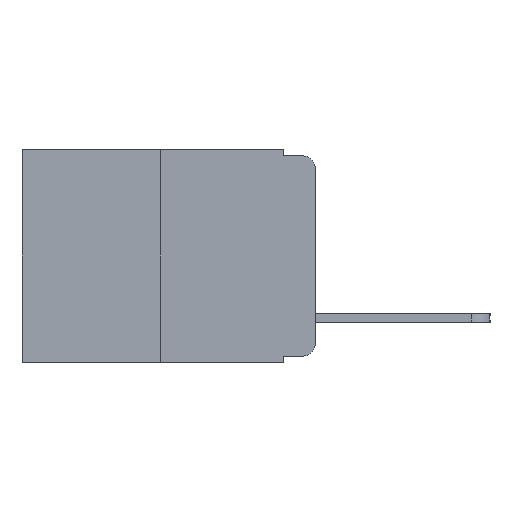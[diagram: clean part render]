
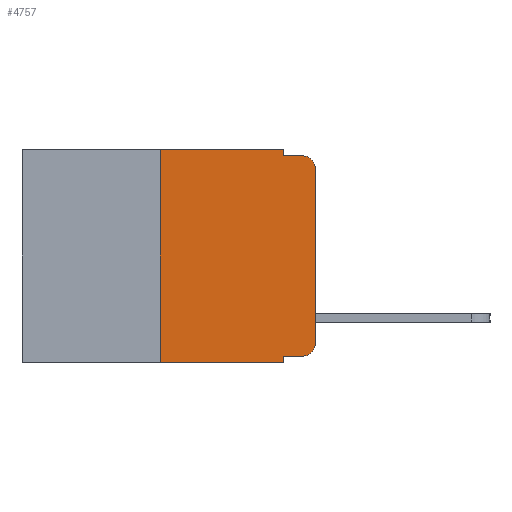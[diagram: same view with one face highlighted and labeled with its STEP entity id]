
A CAD part, left-side view. The second image highlights one B-rep face of the part: STEP entity #4757.
In plain terms, the highlighted planar face has unit normal (-1, 0, 0).
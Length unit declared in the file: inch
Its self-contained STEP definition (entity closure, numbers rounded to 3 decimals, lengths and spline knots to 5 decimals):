
#503 = VERTEX_POINT ( 'NONE', #1208 ) ;
#632 = DIRECTION ( 'NONE',  ( 0., 0., -1. ) ) ;
#1208 = CARTESIAN_POINT ( 'NONE',  ( 0., 0., -0.313 ) ) ;
#1464 = DIRECTION ( 'NONE',  ( 0., -1., 0. ) ) ;
#1510 = VECTOR ( 'NONE', #7378, 39.37008 ) ;
#1657 = LINE ( 'NONE', #4870, #13561 ) ;
#1667 = AXIS2_PLACEMENT_3D ( 'NONE', #4484, #5645, #13725 ) ;
#1835 = AXIS2_PLACEMENT_3D ( 'NONE', #14450, #7539, #632 ) ;
#2133 = CIRCLE ( 'NONE', #3770, 0.02 ) ;
#2329 = EDGE_CURVE ( 'NONE', #2758, #6144, #1657, .T. ) ;
#2381 = VECTOR ( 'NONE', #5413, 39.37008 ) ;
#2434 = EDGE_CURVE ( 'NONE', #12145, #6104, #10714, .T. ) ;
#2583 = EDGE_CURVE ( 'NONE', #11975, #2758, #11249, .T. ) ;
#2726 = ORIENTED_EDGE ( 'NONE', *, *, #2434, .F. ) ;
#2758 = VERTEX_POINT ( 'NONE', #14878 ) ;
#2900 = VERTEX_POINT ( 'NONE', #10627 ) ;
#3063 = EDGE_CURVE ( 'NONE', #3252, #11975, #4716, .T. ) ;
#3070 = EDGE_LOOP ( 'NONE', ( #3589, #12847, #13886, #4369, #11630, #12729, #10726, #2726, #9956, #5263 ) ) ;
#3252 = VERTEX_POINT ( 'NONE', #11225 ) ;
#3296 = CARTESIAN_POINT ( 'NONE',  ( 0., 0.051, -0.333 ) ) ;
#3589 = ORIENTED_EDGE ( 'NONE', *, *, #11612, .T. ) ;
#3770 = AXIS2_PLACEMENT_3D ( 'NONE', #13315, #6368, #14443 ) ;
#3987 = CARTESIAN_POINT ( 'NONE',  ( 0., 0.473, 0. ) ) ;
#4195 = EDGE_CURVE ( 'NONE', #12145, #2900, #8632, .T. ) ;
#4244 = CARTESIAN_POINT ( 'NONE',  ( 0., 0.051, 0. ) ) ;
#4254 = EDGE_CURVE ( 'NONE', #2900, #503, #2133, .T. ) ;
#4369 = ORIENTED_EDGE ( 'NONE', *, *, #2583, .F. ) ;
#4417 = EDGE_CURVE ( 'NONE', #7759, #6104, #14564, .T. ) ;
#4463 = FACE_OUTER_BOUND ( 'NONE', #3070, .T. ) ;
#4484 = CARTESIAN_POINT ( 'NONE',  ( 0., 0.473, 0. ) ) ;
#4716 = LINE ( 'NONE', #3987, #13564 ) ;
#4757 = ADVANCED_FACE ( 'NONE', ( #4463 ), #11435, .F. ) ;
#4759 = CARTESIAN_POINT ( 'NONE',  ( 0., 0.051, -0.343 ) ) ;
#4870 = CARTESIAN_POINT ( 'NONE',  ( 0., 0.051, -0.01 ) ) ;
#4887 = CARTESIAN_POINT ( 'NONE',  ( 0., 0.25, 0. ) ) ;
#4995 = EDGE_CURVE ( 'NONE', #7759, #3252, #12805, .T. ) ;
#5147 = DIRECTION ( 'NONE',  ( 0., -1., 0. ) ) ;
#5263 = ORIENTED_EDGE ( 'NONE', *, *, #4254, .T. ) ;
#5275 = CARTESIAN_POINT ( 'NONE',  ( 0., 0.051, 0. ) ) ;
#5372 = VECTOR ( 'NONE', #14731, 39.37008 ) ;
#5413 = DIRECTION ( 'NONE',  ( 0., 0., -1. ) ) ;
#5645 = DIRECTION ( 'NONE',  ( 1., 0., 0. ) ) ;
#5792 = DIRECTION ( 'NONE',  ( 0., 0., 1. ) ) ;
#6104 = VERTEX_POINT ( 'NONE', #4759 ) ;
#6144 = VERTEX_POINT ( 'NONE', #7124 ) ;
#6368 = DIRECTION ( 'NONE',  ( -1., 0., 0. ) ) ;
#7124 = CARTESIAN_POINT ( 'NONE',  ( 0., 0.02, -0.01 ) ) ;
#7378 = DIRECTION ( 'NONE',  ( 0., 0., -1. ) ) ;
#7539 = DIRECTION ( 'NONE',  ( -1., 0., 0. ) ) ;
#7759 = VERTEX_POINT ( 'NONE', #7926 ) ;
#7835 = VECTOR ( 'NONE', #5792, 39.37008 ) ;
#7926 = CARTESIAN_POINT ( 'NONE',  ( 0., 0.25, -0.343 ) ) ;
#8284 = VECTOR ( 'NONE', #13221, 39.37008 ) ;
#8632 = LINE ( 'NONE', #12024, #8284 ) ;
#9328 = VECTOR ( 'NONE', #10658, 39.37008 ) ;
#9700 = CARTESIAN_POINT ( 'NONE',  ( 0., 0.051, 0. ) ) ;
#9956 = ORIENTED_EDGE ( 'NONE', *, *, #4195, .T. ) ;
#10401 = CARTESIAN_POINT ( 'NONE',  ( 0., 0., 0. ) ) ;
#10627 = CARTESIAN_POINT ( 'NONE',  ( 0., 0.02, -0.333 ) ) ;
#10638 = CARTESIAN_POINT ( 'NONE',  ( 0., 0., -0.03 ) ) ;
#10658 = DIRECTION ( 'NONE',  ( 0., 0., 1. ) ) ;
#10714 = LINE ( 'NONE', #9700, #1510 ) ;
#10726 = ORIENTED_EDGE ( 'NONE', *, *, #4417, .T. ) ;
#10918 = LINE ( 'NONE', #10401, #7835 ) ;
#11225 = CARTESIAN_POINT ( 'NONE',  ( 0., 0.25, 0. ) ) ;
#11249 = LINE ( 'NONE', #4244, #2381 ) ;
#11435 = PLANE ( 'NONE',  #1667 ) ;
#11612 = EDGE_CURVE ( 'NONE', #503, #14198, #10918, .T. ) ;
#11630 = ORIENTED_EDGE ( 'NONE', *, *, #3063, .F. ) ;
#11939 = EDGE_CURVE ( 'NONE', #14198, #6144, #13086, .T. ) ;
#11975 = VERTEX_POINT ( 'NONE', #5275 ) ;
#12024 = CARTESIAN_POINT ( 'NONE',  ( 0., 0.051, -0.333 ) ) ;
#12145 = VERTEX_POINT ( 'NONE', #3296 ) ;
#12729 = ORIENTED_EDGE ( 'NONE', *, *, #4995, .F. ) ;
#12805 = LINE ( 'NONE', #4887, #9328 ) ;
#12847 = ORIENTED_EDGE ( 'NONE', *, *, #11939, .T. ) ;
#13086 = CIRCLE ( 'NONE', #1835, 0.02 ) ;
#13221 = DIRECTION ( 'NONE',  ( 0., -1., 0. ) ) ;
#13315 = CARTESIAN_POINT ( 'NONE',  ( 0., 0.02, -0.313 ) ) ;
#13561 = VECTOR ( 'NONE', #1464, 39.37008 ) ;
#13564 = VECTOR ( 'NONE', #5147, 39.37008 ) ;
#13603 = CARTESIAN_POINT ( 'NONE',  ( 0., 0.473, -0.343 ) ) ;
#13725 = DIRECTION ( 'NONE',  ( 0., 0., -1. ) ) ;
#13886 = ORIENTED_EDGE ( 'NONE', *, *, #2329, .F. ) ;
#14198 = VERTEX_POINT ( 'NONE', #10638 ) ;
#14443 = DIRECTION ( 'NONE',  ( 0., 0., -1. ) ) ;
#14450 = CARTESIAN_POINT ( 'NONE',  ( 0., 0.02, -0.03 ) ) ;
#14564 = LINE ( 'NONE', #13603, #5372 ) ;
#14731 = DIRECTION ( 'NONE',  ( 0., -1., 0. ) ) ;
#14878 = CARTESIAN_POINT ( 'NONE',  ( 0., 0.051, -0.01 ) ) ;
